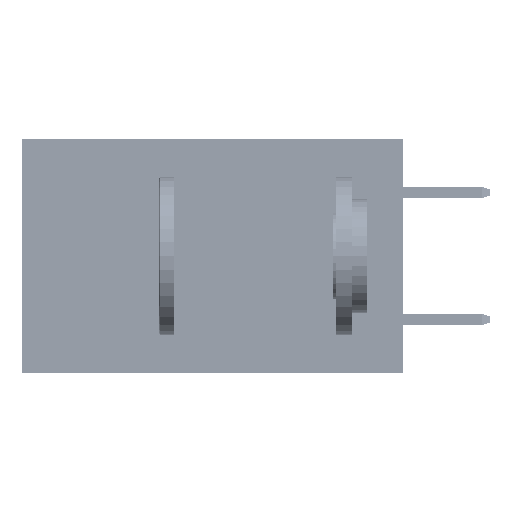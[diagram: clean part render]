
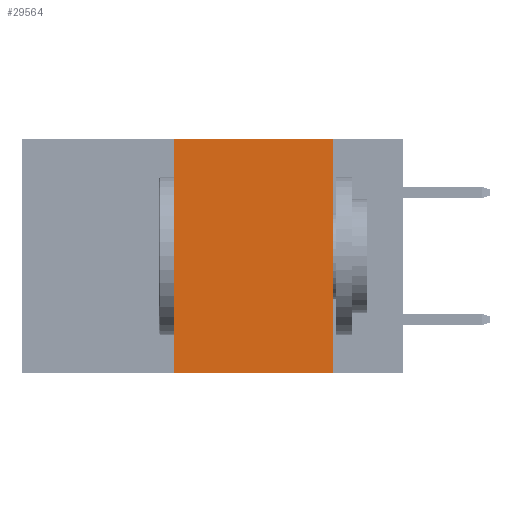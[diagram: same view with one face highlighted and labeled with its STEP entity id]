
A CAD part, left-side view. The second image highlights one B-rep face of the part: STEP entity #29564.
In plain terms, the highlighted planar face has unit normal (-1, 0, 0).
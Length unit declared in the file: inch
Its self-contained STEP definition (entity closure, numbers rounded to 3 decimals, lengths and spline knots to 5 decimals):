
#1736 = DIRECTION ( 'NONE',  ( 0., 0., -1. ) ) ;
#3357 = DIRECTION ( 'NONE',  ( 1., 0., 0. ) ) ;
#5820 = CARTESIAN_POINT ( 'NONE',  ( 0., 0.36, 0. ) ) ;
#6496 = DIRECTION ( 'NONE',  ( 0., -1., 0. ) ) ;
#6958 = CARTESIAN_POINT ( 'NONE',  ( 0., 0.6, 0. ) ) ;
#9026 = CARTESIAN_POINT ( 'NONE',  ( 0., 0.6, -0.37 ) ) ;
#10537 = CARTESIAN_POINT ( 'NONE',  ( 0., 0.36, -0.37 ) ) ;
#10860 = ORIENTED_EDGE ( 'NONE', *, *, #35530, .T. ) ;
#12892 = LINE ( 'NONE', #9026, #27553 ) ;
#13043 = EDGE_CURVE ( 'NONE', #46457, #21859, #29213, .T. ) ;
#14522 = VERTEX_POINT ( 'NONE', #10537 ) ;
#15053 = ORIENTED_EDGE ( 'NONE', *, *, #13043, .F. ) ;
#19362 = VECTOR ( 'NONE', #1736, 39.37008 ) ;
#20763 = CARTESIAN_POINT ( 'NONE',  ( 0., 0.11, 0. ) ) ;
#21813 = EDGE_CURVE ( 'NONE', #30541, #46457, #49146, .T. ) ;
#21859 = VERTEX_POINT ( 'NONE', #22399 ) ;
#22399 = CARTESIAN_POINT ( 'NONE',  ( 0., 0.11, -0.37 ) ) ;
#22990 = VECTOR ( 'NONE', #34504, 39.37008 ) ;
#25351 = VECTOR ( 'NONE', #6496, 39.37008 ) ;
#27176 = EDGE_CURVE ( 'NONE', #14522, #30541, #34754, .T. ) ;
#27553 = VECTOR ( 'NONE', #28259, 39.37008 ) ;
#28259 = DIRECTION ( 'NONE',  ( 0., -1., 0. ) ) ;
#28783 = AXIS2_PLACEMENT_3D ( 'NONE', #6958, #3357, #28860 ) ;
#28860 = DIRECTION ( 'NONE',  ( 0., 0., -1. ) ) ;
#29213 = LINE ( 'NONE', #20763, #19362 ) ;
#29564 = ADVANCED_FACE ( 'NONE', ( #37077 ), #30305, .F. ) ;
#30141 = CARTESIAN_POINT ( 'NONE',  ( 0., 0.36, 0. ) ) ;
#30305 = PLANE ( 'NONE',  #28783 ) ;
#30541 = VERTEX_POINT ( 'NONE', #5820 ) ;
#31210 = CARTESIAN_POINT ( 'NONE',  ( 0., 0.11, 0. ) ) ;
#32709 = ORIENTED_EDGE ( 'NONE', *, *, #27176, .F. ) ;
#34206 = CARTESIAN_POINT ( 'NONE',  ( 0., 0.6, 0. ) ) ;
#34504 = DIRECTION ( 'NONE',  ( 0., 0., 1. ) ) ;
#34754 = LINE ( 'NONE', #30141, #22990 ) ;
#35530 = EDGE_CURVE ( 'NONE', #14522, #21859, #12892, .T. ) ;
#37077 = FACE_OUTER_BOUND ( 'NONE', #41064, .T. ) ;
#41064 = EDGE_LOOP ( 'NONE', ( #15053, #49482, #32709, #10860 ) ) ;
#46457 = VERTEX_POINT ( 'NONE', #31210 ) ;
#49146 = LINE ( 'NONE', #34206, #25351 ) ;
#49482 = ORIENTED_EDGE ( 'NONE', *, *, #21813, .F. ) ;
